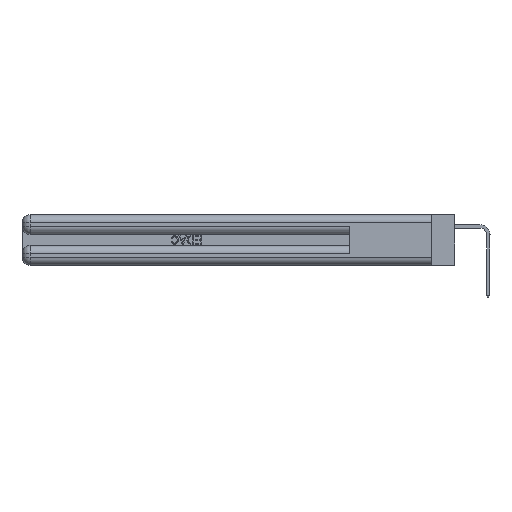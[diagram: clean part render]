
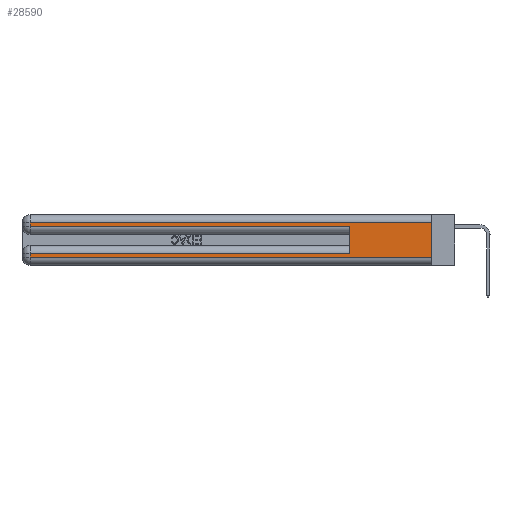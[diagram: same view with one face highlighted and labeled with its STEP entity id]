
A CAD part, left-side view. The second image highlights one B-rep face of the part: STEP entity #28590.
In plain terms, the highlighted planar face has unit normal (-1, 0, 0).
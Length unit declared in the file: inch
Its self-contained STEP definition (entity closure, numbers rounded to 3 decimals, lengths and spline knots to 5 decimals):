
#530 = LINE ( 'NONE', #7961, #25375 ) ;
#785 = CARTESIAN_POINT ( 'NONE',  ( 0., 0., 0.31 ) ) ;
#1157 = DIRECTION ( 'NONE',  ( 0., 0., -1. ) ) ;
#1870 = ORIENTED_EDGE ( 'NONE', *, *, #16106, .T. ) ;
#2245 = CARTESIAN_POINT ( 'NONE',  ( 0., 2.94, 0.06 ) ) ;
#3262 = CARTESIAN_POINT ( 'NONE',  ( 0., 0., 0.085 ) ) ;
#5251 = VECTOR ( 'NONE', #23125, 39.37008 ) ;
#6216 = ORIENTED_EDGE ( 'NONE', *, *, #25670, .T. ) ;
#6521 = CARTESIAN_POINT ( 'NONE',  ( 0., 0.6, 0.145 ) ) ;
#7227 = LINE ( 'NONE', #6521, #24537 ) ;
#7605 = CARTESIAN_POINT ( 'NONE',  ( 0., 0., 0.37 ) ) ;
#7961 = CARTESIAN_POINT ( 'NONE',  ( 0., 0., 0.06 ) ) ;
#10107 = VERTEX_POINT ( 'NONE', #16005 ) ;
#11066 = VECTOR ( 'NONE', #18461, 39.37008 ) ;
#13309 = EDGE_CURVE ( 'NONE', #40781, #36903, #13840, .T. ) ;
#13435 = EDGE_CURVE ( 'NONE', #27232, #23605, #25064, .T. ) ;
#13697 = CARTESIAN_POINT ( 'NONE',  ( 0., 2.94, 0.31 ) ) ;
#13840 = LINE ( 'NONE', #29524, #5251 ) ;
#16005 = CARTESIAN_POINT ( 'NONE',  ( 0., 2.94, 0.085 ) ) ;
#16106 = EDGE_CURVE ( 'NONE', #32384, #23605, #530, .T. ) ;
#16107 = VECTOR ( 'NONE', #18754, 39.37008 ) ;
#17316 = CARTESIAN_POINT ( 'NONE',  ( 0., 0., 0.37 ) ) ;
#17874 = CARTESIAN_POINT ( 'NONE',  ( 0., 0., 0.06 ) ) ;
#18039 = LINE ( 'NONE', #3262, #25674 ) ;
#18461 = DIRECTION ( 'NONE',  ( 0., -1., 0. ) ) ;
#18754 = DIRECTION ( 'NONE',  ( 0., 0., -1. ) ) ;
#19398 = AXIS2_PLACEMENT_3D ( 'NONE', #17316, #40021, #20640 ) ;
#19462 = DIRECTION ( 'NONE',  ( 0., 0., 1. ) ) ;
#19749 = LINE ( 'NONE', #41141, #11066 ) ;
#20422 = VERTEX_POINT ( 'NONE', #33291 ) ;
#20640 = DIRECTION ( 'NONE',  ( 0., 0., -1. ) ) ;
#21358 = ORIENTED_EDGE ( 'NONE', *, *, #40137, .F. ) ;
#21368 = ORIENTED_EDGE ( 'NONE', *, *, #28012, .T. ) ;
#22838 = EDGE_LOOP ( 'NONE', ( #28347, #21368, #40668, #6216, #21358, #23177, #36051, #1870 ) ) ;
#22849 = DIRECTION ( 'NONE',  ( 0., 1., 0. ) ) ;
#23125 = DIRECTION ( 'NONE',  ( 0., 0., -1. ) ) ;
#23177 = ORIENTED_EDGE ( 'NONE', *, *, #27756, .T. ) ;
#23605 = VERTEX_POINT ( 'NONE', #17874 ) ;
#24251 = CARTESIAN_POINT ( 'NONE',  ( 0., 0., 0.31 ) ) ;
#24537 = VECTOR ( 'NONE', #19462, 39.37008 ) ;
#25064 = LINE ( 'NONE', #7605, #33674 ) ;
#25375 = VECTOR ( 'NONE', #33968, 39.37008 ) ;
#25444 = CARTESIAN_POINT ( 'NONE',  ( 0., 2.94, 0.37 ) ) ;
#25670 = EDGE_CURVE ( 'NONE', #36903, #20422, #19749, .T. ) ;
#25674 = VECTOR ( 'NONE', #22849, 39.37008 ) ;
#27232 = VERTEX_POINT ( 'NONE', #785 ) ;
#27756 = EDGE_CURVE ( 'NONE', #31261, #10107, #18039, .T. ) ;
#28012 = EDGE_CURVE ( 'NONE', #27232, #40781, #33776, .T. ) ;
#28347 = ORIENTED_EDGE ( 'NONE', *, *, #13435, .F. ) ;
#28590 = ADVANCED_FACE ( 'NONE', ( #28676 ), #33518, .F. ) ;
#28676 = FACE_OUTER_BOUND ( 'NONE', #22838, .T. ) ;
#29524 = CARTESIAN_POINT ( 'NONE',  ( 0., 2.94, 0.37 ) ) ;
#30188 = CARTESIAN_POINT ( 'NONE',  ( 0., 2.94, 0.285 ) ) ;
#31261 = VERTEX_POINT ( 'NONE', #33941 ) ;
#32384 = VERTEX_POINT ( 'NONE', #2245 ) ;
#32750 = VECTOR ( 'NONE', #37124, 39.37008 ) ;
#33291 = CARTESIAN_POINT ( 'NONE',  ( 0., 0.6, 0.285 ) ) ;
#33430 = LINE ( 'NONE', #25444, #16107 ) ;
#33518 = PLANE ( 'NONE',  #19398 ) ;
#33674 = VECTOR ( 'NONE', #1157, 39.37008 ) ;
#33776 = LINE ( 'NONE', #24251, #32750 ) ;
#33941 = CARTESIAN_POINT ( 'NONE',  ( 0., 0.6, 0.085 ) ) ;
#33968 = DIRECTION ( 'NONE',  ( 0., -1., 0. ) ) ;
#36051 = ORIENTED_EDGE ( 'NONE', *, *, #37285, .T. ) ;
#36903 = VERTEX_POINT ( 'NONE', #30188 ) ;
#37124 = DIRECTION ( 'NONE',  ( 0., 1., 0. ) ) ;
#37285 = EDGE_CURVE ( 'NONE', #10107, #32384, #33430, .T. ) ;
#40021 = DIRECTION ( 'NONE',  ( 1., 0., 0. ) ) ;
#40137 = EDGE_CURVE ( 'NONE', #31261, #20422, #7227, .T. ) ;
#40668 = ORIENTED_EDGE ( 'NONE', *, *, #13309, .T. ) ;
#40781 = VERTEX_POINT ( 'NONE', #13697 ) ;
#41141 = CARTESIAN_POINT ( 'NONE',  ( 0., 0., 0.285 ) ) ;
